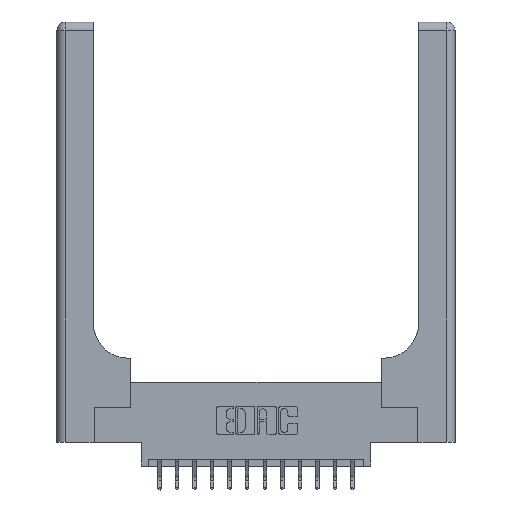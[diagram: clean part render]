
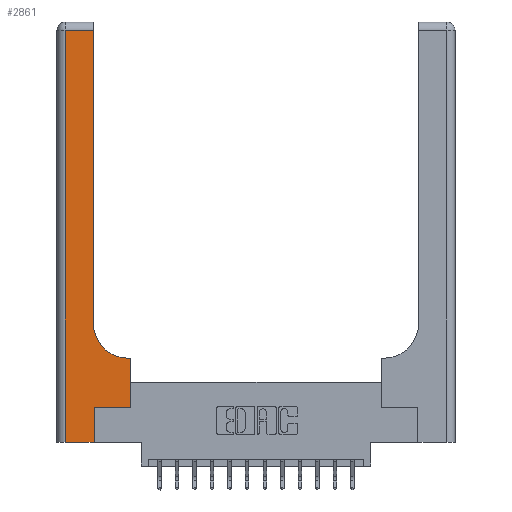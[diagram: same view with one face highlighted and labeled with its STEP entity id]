
A CAD part, top view. The second image highlights one B-rep face of the part: STEP entity #2861.
In plain terms, the highlighted planar face has unit normal (0, 0, 1).
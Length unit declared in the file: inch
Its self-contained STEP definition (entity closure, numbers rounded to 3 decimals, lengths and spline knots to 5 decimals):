
#214 = CARTESIAN_POINT ( 'NONE',  ( 0.528, 0.25, 0.37 ) ) ;
#259 = LINE ( 'NONE', #15019, #10660 ) ;
#509 = DIRECTION ( 'NONE',  ( 1., 0., 0. ) ) ;
#1572 = DIRECTION ( 'NONE',  ( -1., 0., 0. ) ) ;
#1640 = VERTEX_POINT ( 'NONE', #5691 ) ;
#2130 = FACE_OUTER_BOUND ( 'NONE', #3513, .T. ) ;
#2481 = ORIENTED_EDGE ( 'NONE', *, *, #16723, .T. ) ;
#2546 = DIRECTION ( 'NONE',  ( -1., 0., 0. ) ) ;
#2573 = VERTEX_POINT ( 'NONE', #12676 ) ;
#2772 = EDGE_CURVE ( 'NONE', #6326, #1640, #2963, .T. ) ;
#2861 = ADVANCED_FACE ( 'NONE', ( #2130 ), #17270, .F. ) ;
#2963 = LINE ( 'NONE', #5123, #3400 ) ;
#3198 = VERTEX_POINT ( 'NONE', #4564 ) ;
#3204 = EDGE_CURVE ( 'NONE', #2573, #3405, #7428, .T. ) ;
#3400 = VECTOR ( 'NONE', #14463, 39.37008 ) ;
#3405 = VERTEX_POINT ( 'NONE', #14268 ) ;
#3461 = EDGE_CURVE ( 'NONE', #7445, #10354, #10093, .T. ) ;
#3513 = EDGE_LOOP ( 'NONE', ( #3583, #2481, #11892, #4459, #10560, #7345, #4744, #12461, #7583 ) ) ;
#3583 = ORIENTED_EDGE ( 'NONE', *, *, #2772, .T. ) ;
#3728 = CARTESIAN_POINT ( 'NONE',  ( 0., 0., 0.37 ) ) ;
#4403 = AXIS2_PLACEMENT_3D ( 'NONE', #13169, #5169, #14501 ) ;
#4459 = ORIENTED_EDGE ( 'NONE', *, *, #3461, .T. ) ;
#4564 = CARTESIAN_POINT ( 'NONE',  ( 0.51, 0.6, 0.37 ) ) ;
#4744 = ORIENTED_EDGE ( 'NONE', *, *, #6217, .T. ) ;
#4914 = LINE ( 'NONE', #214, #5356 ) ;
#4937 = CARTESIAN_POINT ( 'NONE',  ( 0.26, 0.6, 0.37 ) ) ;
#5123 = CARTESIAN_POINT ( 'NONE',  ( 0.26, 3., 0.37 ) ) ;
#5169 = DIRECTION ( 'NONE',  ( 0., 0., -1. ) ) ;
#5356 = VECTOR ( 'NONE', #9717, 39.37008 ) ;
#5668 = VERTEX_POINT ( 'NONE', #16339 ) ;
#5691 = CARTESIAN_POINT ( 'NONE',  ( 0.26, 2.94, 0.37 ) ) ;
#6079 = CARTESIAN_POINT ( 'NONE',  ( 0.06, 2.94, 0.37 ) ) ;
#6217 = EDGE_CURVE ( 'NONE', #3405, #5668, #4914, .T. ) ;
#6326 = VERTEX_POINT ( 'NONE', #13811 ) ;
#6506 = VECTOR ( 'NONE', #15792, 39.37008 ) ;
#7295 = LINE ( 'NONE', #9690, #10856 ) ;
#7345 = ORIENTED_EDGE ( 'NONE', *, *, #3204, .T. ) ;
#7428 = LINE ( 'NONE', #10011, #14912 ) ;
#7445 = VERTEX_POINT ( 'NONE', #10782 ) ;
#7583 = ORIENTED_EDGE ( 'NONE', *, *, #14203, .T. ) ;
#8408 = CIRCLE ( 'NONE', #4403, 0.25 ) ;
#8979 = LINE ( 'NONE', #9154, #16032 ) ;
#9154 = CARTESIAN_POINT ( 'NONE',  ( 0.265, 0., 0.37 ) ) ;
#9309 = CARTESIAN_POINT ( 'NONE',  ( 0., 3., 0.37 ) ) ;
#9690 = CARTESIAN_POINT ( 'NONE',  ( 0., 2.94, 0.37 ) ) ;
#9717 = DIRECTION ( 'NONE',  ( 0., 1., 0. ) ) ;
#9856 = VECTOR ( 'NONE', #11678, 39.37008 ) ;
#10011 = CARTESIAN_POINT ( 'NONE',  ( 0.265, 0.25, 0.37 ) ) ;
#10093 = LINE ( 'NONE', #3728, #6506 ) ;
#10280 = LINE ( 'NONE', #4937, #9856 ) ;
#10354 = VERTEX_POINT ( 'NONE', #10873 ) ;
#10515 = DIRECTION ( 'NONE',  ( 0., 1., 0. ) ) ;
#10560 = ORIENTED_EDGE ( 'NONE', *, *, #17157, .T. ) ;
#10659 = DIRECTION ( 'NONE',  ( 0., 0., -1. ) ) ;
#10660 = VECTOR ( 'NONE', #16357, 39.37008 ) ;
#10782 = CARTESIAN_POINT ( 'NONE',  ( 0.06, 0., 0.37 ) ) ;
#10856 = VECTOR ( 'NONE', #1572, 39.37008 ) ;
#10873 = CARTESIAN_POINT ( 'NONE',  ( 0.265, 0., 0.37 ) ) ;
#11678 = DIRECTION ( 'NONE',  ( -1., 0., 0. ) ) ;
#11776 = VERTEX_POINT ( 'NONE', #6079 ) ;
#11842 = EDGE_CURVE ( 'NONE', #5668, #3198, #10280, .T. ) ;
#11892 = ORIENTED_EDGE ( 'NONE', *, *, #12712, .T. ) ;
#12461 = ORIENTED_EDGE ( 'NONE', *, *, #11842, .T. ) ;
#12676 = CARTESIAN_POINT ( 'NONE',  ( 0.265, 0.25, 0.37 ) ) ;
#12712 = EDGE_CURVE ( 'NONE', #11776, #7445, #259, .T. ) ;
#13169 = CARTESIAN_POINT ( 'NONE',  ( 0.51, 0.85, 0.37 ) ) ;
#13811 = CARTESIAN_POINT ( 'NONE',  ( 0.26, 0.85, 0.37 ) ) ;
#13993 = AXIS2_PLACEMENT_3D ( 'NONE', #9309, #10659, #2546 ) ;
#14203 = EDGE_CURVE ( 'NONE', #3198, #6326, #8408, .T. ) ;
#14268 = CARTESIAN_POINT ( 'NONE',  ( 0.528, 0.25, 0.37 ) ) ;
#14463 = DIRECTION ( 'NONE',  ( 0., 1., 0. ) ) ;
#14501 = DIRECTION ( 'NONE',  ( 1., 0., 0. ) ) ;
#14912 = VECTOR ( 'NONE', #509, 39.37008 ) ;
#15019 = CARTESIAN_POINT ( 'NONE',  ( 0.06, 3., 0.37 ) ) ;
#15792 = DIRECTION ( 'NONE',  ( 1., 0., 0. ) ) ;
#16032 = VECTOR ( 'NONE', #10515, 39.37008 ) ;
#16339 = CARTESIAN_POINT ( 'NONE',  ( 0.528, 0.6, 0.37 ) ) ;
#16357 = DIRECTION ( 'NONE',  ( 0., -1., 0. ) ) ;
#16723 = EDGE_CURVE ( 'NONE', #1640, #11776, #7295, .T. ) ;
#17157 = EDGE_CURVE ( 'NONE', #10354, #2573, #8979, .T. ) ;
#17270 = PLANE ( 'NONE',  #13993 ) ;
